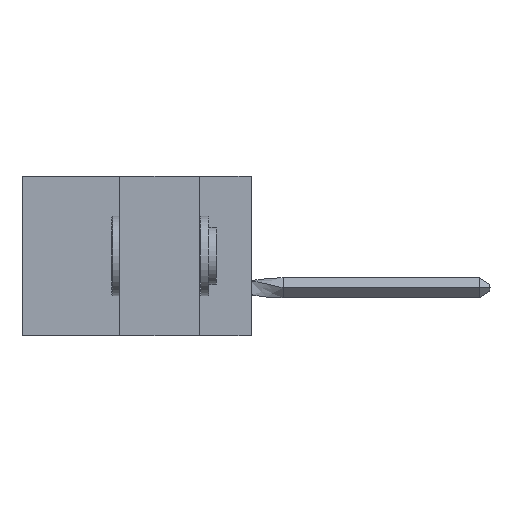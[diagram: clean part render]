
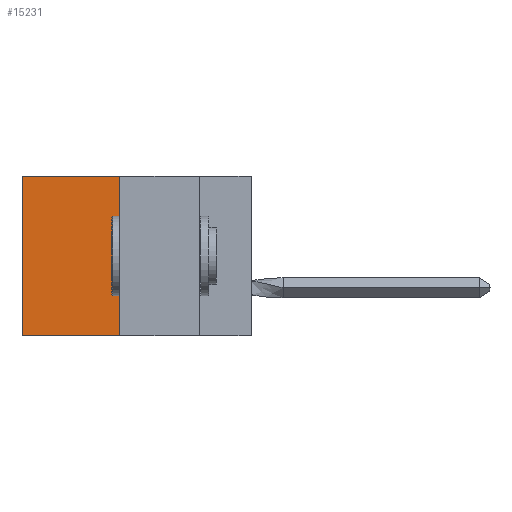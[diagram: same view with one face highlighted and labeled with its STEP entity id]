
A CAD part, left-side view. The second image highlights one B-rep face of the part: STEP entity #15231.
In plain terms, the highlighted planar face has unit normal (-1, 0, 0).
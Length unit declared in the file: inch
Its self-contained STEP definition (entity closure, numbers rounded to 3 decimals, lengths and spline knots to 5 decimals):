
#290 = VERTEX_POINT ( 'NONE', #8998 ) ;
#721 = LINE ( 'NONE', #4416, #12885 ) ;
#1426 = CARTESIAN_POINT ( 'NONE',  ( 0.305, 0.72, 0. ) ) ;
#1522 = VERTEX_POINT ( 'NONE', #11486 ) ;
#1581 = VECTOR ( 'NONE', #16116, 39.37008 ) ;
#2308 = EDGE_CURVE ( 'NONE', #14189, #1522, #721, .T. ) ;
#2886 = CARTESIAN_POINT ( 'NONE',  ( 0.305, 0.413, -0.5 ) ) ;
#2988 = LINE ( 'NONE', #7281, #11028 ) ;
#4211 = DIRECTION ( 'NONE',  ( 1., 0., 0. ) ) ;
#4416 = CARTESIAN_POINT ( 'NONE',  ( 0.305, 0.413, -0.5 ) ) ;
#5263 = DIRECTION ( 'NONE',  ( 0., 0., -1. ) ) ;
#7281 = CARTESIAN_POINT ( 'NONE',  ( 0.305, 0.72, -0.5 ) ) ;
#7326 = DIRECTION ( 'NONE',  ( 0., 0., -1. ) ) ;
#8090 = CARTESIAN_POINT ( 'NONE',  ( 0.305, 0.413, 0. ) ) ;
#8101 = FACE_OUTER_BOUND ( 'NONE', #8288, .T. ) ;
#8125 = DIRECTION ( 'NONE',  ( 0., 0., -1. ) ) ;
#8288 = EDGE_LOOP ( 'NONE', ( #10879, #16763, #11747, #9462 ) ) ;
#8998 = CARTESIAN_POINT ( 'NONE',  ( 0.305, 0.413, 0. ) ) ;
#9462 = ORIENTED_EDGE ( 'NONE', *, *, #12850, .T. ) ;
#9527 = VERTEX_POINT ( 'NONE', #1426 ) ;
#9597 = CARTESIAN_POINT ( 'NONE',  ( 0.305, 0.413, -0.5 ) ) ;
#10366 = AXIS2_PLACEMENT_3D ( 'NONE', #2886, #4211, #8125 ) ;
#10726 = PLANE ( 'NONE',  #10366 ) ;
#10879 = ORIENTED_EDGE ( 'NONE', *, *, #14363, .T. ) ;
#11028 = VECTOR ( 'NONE', #7326, 39.37008 ) ;
#11486 = CARTESIAN_POINT ( 'NONE',  ( 0.305, 0.72, -0.5 ) ) ;
#11747 = ORIENTED_EDGE ( 'NONE', *, *, #14661, .F. ) ;
#11890 = CARTESIAN_POINT ( 'NONE',  ( 0.305, 0.413, -0.5 ) ) ;
#12486 = LINE ( 'NONE', #8090, #1581 ) ;
#12850 = EDGE_CURVE ( 'NONE', #290, #9527, #12486, .T. ) ;
#12885 = VECTOR ( 'NONE', #13479, 39.37008 ) ;
#13479 = DIRECTION ( 'NONE',  ( 0., 1., 0. ) ) ;
#14189 = VERTEX_POINT ( 'NONE', #9597 ) ;
#14363 = EDGE_CURVE ( 'NONE', #9527, #1522, #2988, .T. ) ;
#14661 = EDGE_CURVE ( 'NONE', #290, #14189, #15677, .T. ) ;
#15231 = ADVANCED_FACE ( 'NONE', ( #8101 ), #10726, .F. ) ;
#15466 = VECTOR ( 'NONE', #5263, 39.37008 ) ;
#15677 = LINE ( 'NONE', #11890, #15466 ) ;
#16116 = DIRECTION ( 'NONE',  ( 0., 1., 0. ) ) ;
#16763 = ORIENTED_EDGE ( 'NONE', *, *, #2308, .F. ) ;
